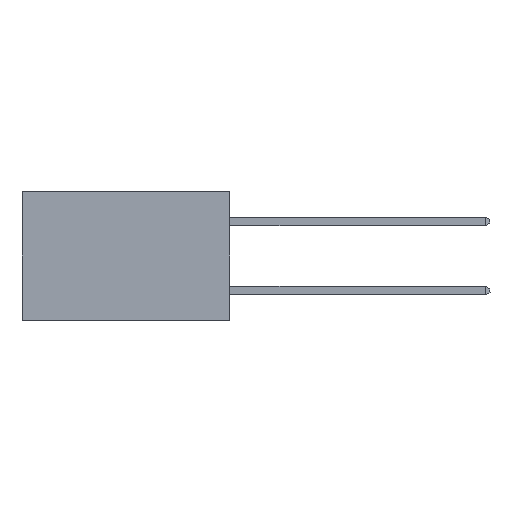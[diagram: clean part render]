
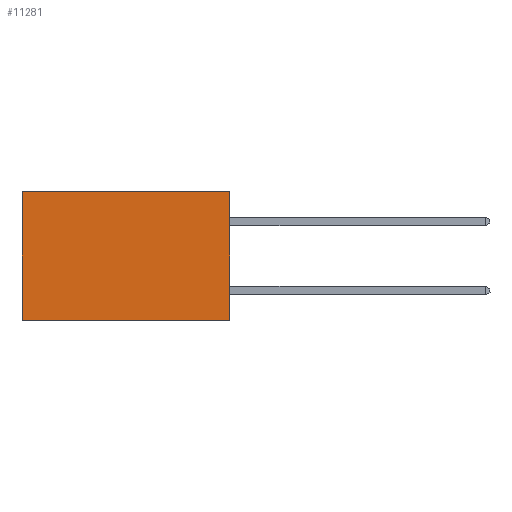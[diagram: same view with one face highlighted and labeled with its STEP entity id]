
A CAD part, left-side view. The second image highlights one B-rep face of the part: STEP entity #11281.
In plain terms, the highlighted planar face has unit normal (-1, 0, 0).
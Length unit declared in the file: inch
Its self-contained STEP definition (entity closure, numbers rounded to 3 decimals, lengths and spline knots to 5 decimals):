
#218 = DIRECTION ( 'NONE',  ( 0., 1., 0. ) ) ;
#350 = DIRECTION ( 'NONE',  ( 1., 0., 0. ) ) ;
#520 = VECTOR ( 'NONE', #13904, 39.37008 ) ;
#1051 = VERTEX_POINT ( 'NONE', #8429 ) ;
#1105 = CARTESIAN_POINT ( 'NONE',  ( 0.298, 0.6, 0. ) ) ;
#2101 = DIRECTION ( 'NONE',  ( 0., 0., -1. ) ) ;
#3009 = CARTESIAN_POINT ( 'NONE',  ( 0.298, 0.6, 0. ) ) ;
#3240 = LINE ( 'NONE', #10216, #520 ) ;
#3787 = EDGE_CURVE ( 'NONE', #1051, #12718, #3240, .T. ) ;
#3876 = DIRECTION ( 'NONE',  ( 0., 0., -1. ) ) ;
#3903 = ORIENTED_EDGE ( 'NONE', *, *, #3787, .T. ) ;
#3970 = AXIS2_PLACEMENT_3D ( 'NONE', #9696, #350, #3876 ) ;
#4186 = FACE_OUTER_BOUND ( 'NONE', #7263, .T. ) ;
#4364 = VERTEX_POINT ( 'NONE', #13119 ) ;
#5527 = VECTOR ( 'NONE', #218, 39.37008 ) ;
#6213 = PLANE ( 'NONE',  #3970 ) ;
#6691 = LINE ( 'NONE', #7051, #12631 ) ;
#7051 = CARTESIAN_POINT ( 'NONE',  ( 0.298, 0., 0. ) ) ;
#7263 = EDGE_LOOP ( 'NONE', ( #9082, #14237, #11646, #3903 ) ) ;
#7699 = CARTESIAN_POINT ( 'NONE',  ( 0.298, 0.6, -0.37 ) ) ;
#7963 = LINE ( 'NONE', #14341, #5527 ) ;
#8026 = EDGE_CURVE ( 'NONE', #12718, #14944, #11389, .T. ) ;
#8271 = DIRECTION ( 'NONE',  ( 0., 0., -1. ) ) ;
#8429 = CARTESIAN_POINT ( 'NONE',  ( 0.298, 0., 0. ) ) ;
#9082 = ORIENTED_EDGE ( 'NONE', *, *, #8026, .T. ) ;
#9359 = VECTOR ( 'NONE', #2101, 39.37008 ) ;
#9696 = CARTESIAN_POINT ( 'NONE',  ( 0.298, 0., 0. ) ) ;
#10216 = CARTESIAN_POINT ( 'NONE',  ( 0.298, 0., 0. ) ) ;
#10463 = EDGE_CURVE ( 'NONE', #4364, #14944, #7963, .T. ) ;
#11281 = ADVANCED_FACE ( 'NONE', ( #4186 ), #6213, .F. ) ;
#11389 = LINE ( 'NONE', #1105, #9359 ) ;
#11646 = ORIENTED_EDGE ( 'NONE', *, *, #15244, .F. ) ;
#12631 = VECTOR ( 'NONE', #8271, 39.37008 ) ;
#12718 = VERTEX_POINT ( 'NONE', #3009 ) ;
#13119 = CARTESIAN_POINT ( 'NONE',  ( 0.298, 0., -0.37 ) ) ;
#13904 = DIRECTION ( 'NONE',  ( 0., 1., 0. ) ) ;
#14237 = ORIENTED_EDGE ( 'NONE', *, *, #10463, .F. ) ;
#14341 = CARTESIAN_POINT ( 'NONE',  ( 0.298, 0., -0.37 ) ) ;
#14944 = VERTEX_POINT ( 'NONE', #7699 ) ;
#15244 = EDGE_CURVE ( 'NONE', #1051, #4364, #6691, .T. ) ;
